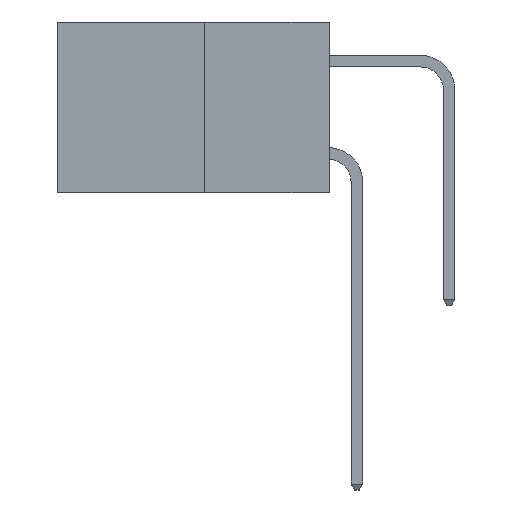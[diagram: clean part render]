
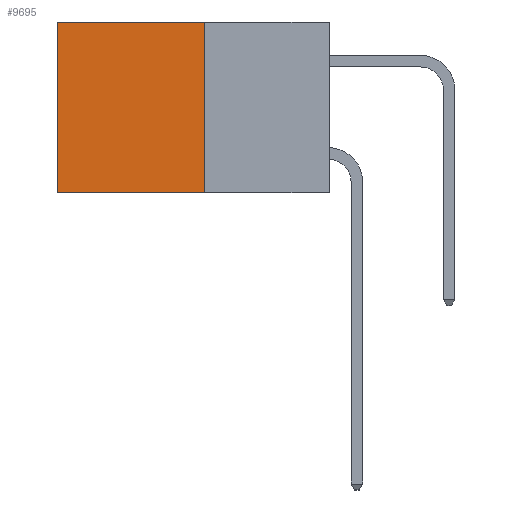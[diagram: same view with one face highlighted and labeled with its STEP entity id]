
A CAD part, left-side view. The second image highlights one B-rep face of the part: STEP entity #9695.
In plain terms, the highlighted planar face has unit normal (-1, 0, 0).
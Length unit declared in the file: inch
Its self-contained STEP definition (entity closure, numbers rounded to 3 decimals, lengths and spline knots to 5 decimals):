
#443 = PLANE ( 'NONE',  #10048 ) ;
#825 = VECTOR ( 'NONE', #8587, 39.37008 ) ;
#1086 = LINE ( 'NONE', #4822, #825 ) ;
#1249 = CARTESIAN_POINT ( 'NONE',  ( 0.277, 0.27, -0.37 ) ) ;
#1753 = DIRECTION ( 'NONE',  ( 0., 0., -1. ) ) ;
#1856 = DIRECTION ( 'NONE',  ( 0., 1., 0. ) ) ;
#2132 = DIRECTION ( 'NONE',  ( 0., 0., -1. ) ) ;
#3005 = VERTEX_POINT ( 'NONE', #6231 ) ;
#3237 = CARTESIAN_POINT ( 'NONE',  ( 0.277, 0.59, 0. ) ) ;
#4320 = VECTOR ( 'NONE', #1856, 39.37008 ) ;
#4735 = EDGE_CURVE ( 'NONE', #9268, #3005, #6169, .T. ) ;
#4822 = CARTESIAN_POINT ( 'NONE',  ( 0.277, 0.27, 0. ) ) ;
#5086 = EDGE_CURVE ( 'NONE', #5848, #9268, #5329, .T. ) ;
#5203 = VECTOR ( 'NONE', #1753, 39.37008 ) ;
#5329 = LINE ( 'NONE', #9252, #9079 ) ;
#5460 = FACE_OUTER_BOUND ( 'NONE', #5787, .T. ) ;
#5787 = EDGE_LOOP ( 'NONE', ( #6700, #6759, #6919, #7140 ) ) ;
#5848 = VERTEX_POINT ( 'NONE', #6684 ) ;
#6164 = CARTESIAN_POINT ( 'NONE',  ( 0.277, 0.27, -0.37 ) ) ;
#6169 = LINE ( 'NONE', #1249, #4320 ) ;
#6231 = CARTESIAN_POINT ( 'NONE',  ( 0.277, 0.59, -0.37 ) ) ;
#6270 = EDGE_CURVE ( 'NONE', #9208, #3005, #7200, .T. ) ;
#6684 = CARTESIAN_POINT ( 'NONE',  ( 0.277, 0.27, 0. ) ) ;
#6700 = ORIENTED_EDGE ( 'NONE', *, *, #6270, .T. ) ;
#6759 = ORIENTED_EDGE ( 'NONE', *, *, #4735, .F. ) ;
#6913 = DIRECTION ( 'NONE',  ( 1., 0., 0. ) ) ;
#6919 = ORIENTED_EDGE ( 'NONE', *, *, #5086, .F. ) ;
#7140 = ORIENTED_EDGE ( 'NONE', *, *, #8079, .T. ) ;
#7200 = LINE ( 'NONE', #9518, #5203 ) ;
#7215 = CARTESIAN_POINT ( 'NONE',  ( 0.277, 0.27, -0.37 ) ) ;
#8079 = EDGE_CURVE ( 'NONE', #5848, #9208, #1086, .T. ) ;
#8587 = DIRECTION ( 'NONE',  ( 0., 1., 0. ) ) ;
#9079 = VECTOR ( 'NONE', #9087, 39.37008 ) ;
#9087 = DIRECTION ( 'NONE',  ( 0., 0., -1. ) ) ;
#9208 = VERTEX_POINT ( 'NONE', #3237 ) ;
#9252 = CARTESIAN_POINT ( 'NONE',  ( 0.277, 0.27, -0.37 ) ) ;
#9268 = VERTEX_POINT ( 'NONE', #7215 ) ;
#9518 = CARTESIAN_POINT ( 'NONE',  ( 0.277, 0.59, -0.37 ) ) ;
#9695 = ADVANCED_FACE ( 'NONE', ( #5460 ), #443, .F. ) ;
#10048 = AXIS2_PLACEMENT_3D ( 'NONE', #6164, #6913, #2132 ) ;
